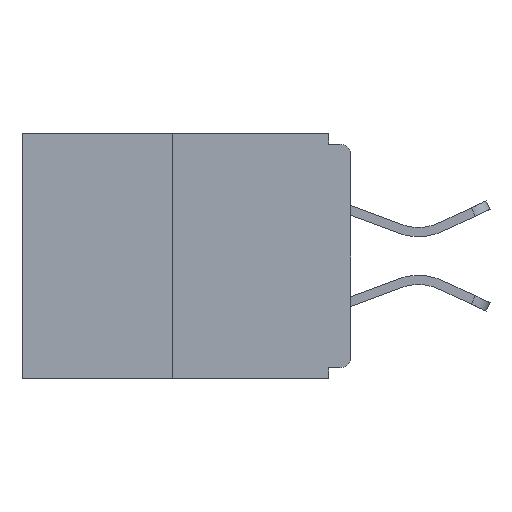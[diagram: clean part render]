
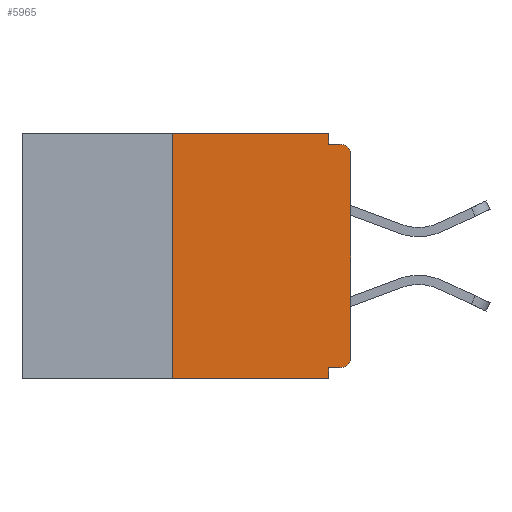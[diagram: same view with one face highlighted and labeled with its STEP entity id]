
A CAD part, left-side view. The second image highlights one B-rep face of the part: STEP entity #5965.
In plain terms, the highlighted planar face has unit normal (-1, 0, 0).
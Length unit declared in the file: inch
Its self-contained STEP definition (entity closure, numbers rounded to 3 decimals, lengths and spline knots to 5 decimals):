
#160 = CARTESIAN_POINT ( 'NONE',  ( 0., 0.031, 0. ) ) ;
#281 = LINE ( 'NONE', #7737, #9474 ) ;
#309 = EDGE_CURVE ( 'NONE', #4915, #6220, #646, .T. ) ;
#416 = EDGE_CURVE ( 'NONE', #12091, #11502, #1184, .T. ) ;
#444 = DIRECTION ( 'NONE',  ( 0., 0., -1. ) ) ;
#614 = DIRECTION ( 'NONE',  ( 1., 0., 0. ) ) ;
#616 = AXIS2_PLACEMENT_3D ( 'NONE', #5116, #7331, #444 ) ;
#646 = LINE ( 'NONE', #12862, #12579 ) ;
#1065 = VERTEX_POINT ( 'NONE', #13293 ) ;
#1113 = CARTESIAN_POINT ( 'NONE',  ( 0., 0., -0.313 ) ) ;
#1148 = CARTESIAN_POINT ( 'NONE',  ( 0., 0.031, 0. ) ) ;
#1184 = CIRCLE ( 'NONE', #5403, 0.015 ) ;
#1432 = VERTEX_POINT ( 'NONE', #6892 ) ;
#1497 = CARTESIAN_POINT ( 'NONE',  ( 0., 0.031, -0.328 ) ) ;
#1508 = CARTESIAN_POINT ( 'NONE',  ( 0., 0.015, -0.313 ) ) ;
#1561 = LINE ( 'NONE', #5027, #5135 ) ;
#1634 = CARTESIAN_POINT ( 'NONE',  ( 0., 0.031, -0.015 ) ) ;
#1930 = EDGE_CURVE ( 'NONE', #1432, #14838, #6354, .T. ) ;
#2536 = CARTESIAN_POINT ( 'NONE',  ( 0., 0.25, 0. ) ) ;
#2630 = DIRECTION ( 'NONE',  ( 0., 1., 0. ) ) ;
#2683 = DIRECTION ( 'NONE',  ( 0., 0., -1. ) ) ;
#2689 = DIRECTION ( 'NONE',  ( 0., 0., 1. ) ) ;
#2757 = EDGE_CURVE ( 'NONE', #1065, #6220, #14280, .T. ) ;
#3250 = ORIENTED_EDGE ( 'NONE', *, *, #2757, .T. ) ;
#3362 = LINE ( 'NONE', #1148, #14744 ) ;
#3398 = VERTEX_POINT ( 'NONE', #1634 ) ;
#3876 = DIRECTION ( 'NONE',  ( 0., 0., -1. ) ) ;
#4901 = ORIENTED_EDGE ( 'NONE', *, *, #309, .F. ) ;
#4915 = VERTEX_POINT ( 'NONE', #1497 ) ;
#4988 = LINE ( 'NONE', #9320, #8967 ) ;
#5027 = CARTESIAN_POINT ( 'NONE',  ( 0., 0., 0. ) ) ;
#5080 = ORIENTED_EDGE ( 'NONE', *, *, #5216, .F. ) ;
#5116 = CARTESIAN_POINT ( 'NONE',  ( 0., 0.015, -0.03 ) ) ;
#5135 = VECTOR ( 'NONE', #7350, 39.37008 ) ;
#5216 = EDGE_CURVE ( 'NONE', #12091, #4915, #4988, .T. ) ;
#5403 = AXIS2_PLACEMENT_3D ( 'NONE', #1508, #11623, #3876 ) ;
#5620 = DIRECTION ( 'NONE',  ( 0., -1., 0. ) ) ;
#5718 = EDGE_CURVE ( 'NONE', #14838, #3398, #3362, .T. ) ;
#5792 = VECTOR ( 'NONE', #5620, 39.37008 ) ;
#5945 = CARTESIAN_POINT ( 'NONE',  ( 0., 0.015, -0.328 ) ) ;
#5965 = ADVANCED_FACE ( 'NONE', ( #6764 ), #13494, .F. ) ;
#6093 = EDGE_CURVE ( 'NONE', #11502, #9491, #1561, .T. ) ;
#6184 = CARTESIAN_POINT ( 'NONE',  ( 0., 0., -0.03 ) ) ;
#6220 = VERTEX_POINT ( 'NONE', #12692 ) ;
#6340 = CARTESIAN_POINT ( 'NONE',  ( 0., 0.46, 0. ) ) ;
#6354 = LINE ( 'NONE', #6340, #12522 ) ;
#6537 = CARTESIAN_POINT ( 'NONE',  ( 0., 0.46, 0. ) ) ;
#6764 = FACE_OUTER_BOUND ( 'NONE', #7423, .T. ) ;
#6892 = CARTESIAN_POINT ( 'NONE',  ( 0., 0.25, 0. ) ) ;
#7108 = VECTOR ( 'NONE', #2689, 39.37008 ) ;
#7331 = DIRECTION ( 'NONE',  ( -1., 0., 0. ) ) ;
#7350 = DIRECTION ( 'NONE',  ( 0., 0., 1. ) ) ;
#7423 = EDGE_LOOP ( 'NONE', ( #14851, #8502, #3250, #4901, #5080, #10954, #8683, #12710, #7834, #10531 ) ) ;
#7461 = CIRCLE ( 'NONE', #616, 0.015 ) ;
#7737 = CARTESIAN_POINT ( 'NONE',  ( 0., 0., -0.015 ) ) ;
#7834 = ORIENTED_EDGE ( 'NONE', *, *, #13007, .F. ) ;
#8502 = ORIENTED_EDGE ( 'NONE', *, *, #11580, .F. ) ;
#8671 = DIRECTION ( 'NONE',  ( 0., 0., -1. ) ) ;
#8683 = ORIENTED_EDGE ( 'NONE', *, *, #6093, .T. ) ;
#8967 = VECTOR ( 'NONE', #2630, 39.37008 ) ;
#9108 = CARTESIAN_POINT ( 'NONE',  ( 0., 0.46, -0.343 ) ) ;
#9320 = CARTESIAN_POINT ( 'NONE',  ( 0., 0., -0.328 ) ) ;
#9474 = VECTOR ( 'NONE', #12362, 39.37008 ) ;
#9491 = VERTEX_POINT ( 'NONE', #6184 ) ;
#9835 = DIRECTION ( 'NONE',  ( 0., -1., 0. ) ) ;
#10356 = CARTESIAN_POINT ( 'NONE',  ( 0., 0.015, -0.015 ) ) ;
#10531 = ORIENTED_EDGE ( 'NONE', *, *, #5718, .F. ) ;
#10820 = VERTEX_POINT ( 'NONE', #10356 ) ;
#10954 = ORIENTED_EDGE ( 'NONE', *, *, #416, .T. ) ;
#11096 = AXIS2_PLACEMENT_3D ( 'NONE', #6537, #614, #8671 ) ;
#11274 = LINE ( 'NONE', #2536, #7108 ) ;
#11502 = VERTEX_POINT ( 'NONE', #1113 ) ;
#11580 = EDGE_CURVE ( 'NONE', #1065, #1432, #11274, .T. ) ;
#11623 = DIRECTION ( 'NONE',  ( -1., 0., 0. ) ) ;
#12091 = VERTEX_POINT ( 'NONE', #5945 ) ;
#12152 = EDGE_CURVE ( 'NONE', #9491, #10820, #7461, .T. ) ;
#12362 = DIRECTION ( 'NONE',  ( 0., -1., 0. ) ) ;
#12522 = VECTOR ( 'NONE', #9835, 39.37008 ) ;
#12579 = VECTOR ( 'NONE', #2683, 39.37008 ) ;
#12692 = CARTESIAN_POINT ( 'NONE',  ( 0., 0.031, -0.343 ) ) ;
#12710 = ORIENTED_EDGE ( 'NONE', *, *, #12152, .T. ) ;
#12862 = CARTESIAN_POINT ( 'NONE',  ( 0., 0.031, -0.343 ) ) ;
#12899 = DIRECTION ( 'NONE',  ( 0., 0., -1. ) ) ;
#13007 = EDGE_CURVE ( 'NONE', #3398, #10820, #281, .T. ) ;
#13293 = CARTESIAN_POINT ( 'NONE',  ( 0., 0.25, -0.343 ) ) ;
#13494 = PLANE ( 'NONE',  #11096 ) ;
#14280 = LINE ( 'NONE', #9108, #5792 ) ;
#14744 = VECTOR ( 'NONE', #12899, 39.37008 ) ;
#14838 = VERTEX_POINT ( 'NONE', #160 ) ;
#14851 = ORIENTED_EDGE ( 'NONE', *, *, #1930, .F. ) ;
